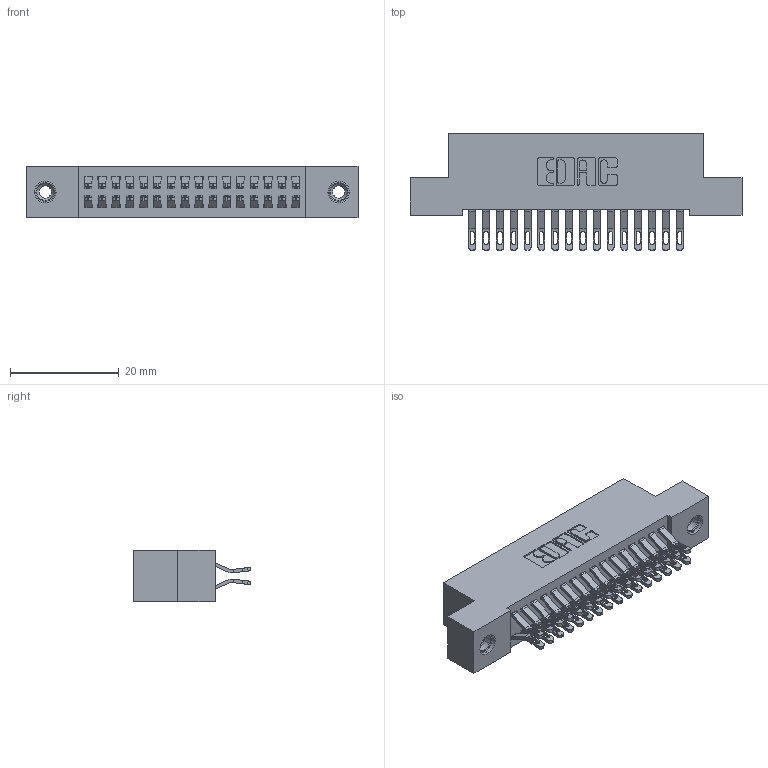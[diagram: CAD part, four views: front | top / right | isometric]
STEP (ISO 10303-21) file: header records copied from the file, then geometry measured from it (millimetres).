
FILE_DESCRIPTION (( 'STEP AP203' ), '1' );
FILE_NAME ('342-032-555-208.STEP', '2018-08-11T17:15:33', ( '' ), ( '' ), 'SwSTEP 2.0', 'SolidWorks 2016', '' );
FILE_SCHEMA (( 'CONFIG_CONTROL_DESIGN' ));
Length unit declared in the file: inch
Products named in the file (4): 342 Part_TI; 345-292-001_555 Tail; 345-250-001_345-250-003-102; 342-032-555-208
Assembly tree (35 placements, depth 2):
  342-032-555-208
    342 Part_TI
    345-292-001_555 Tail  x32
    345-250-001_345-250-003-102  x2
Bounding box: 60.96 x 21.47 x 9.4 mm (x, y, z)
Volume: 5437.4 mm3; surface area: 8530 mm2
Topology: 35 solids, 35 shells, 2026 faces, 6291 edges, 4186 vertices
Faces by surface type: plane 1186, cylinder 824, cone 12, torus 4
Entity records: 15036 total; most frequent: CARTESIAN_POINT 2539, ORIENTED_EDGE 2438, DIRECTION 2217, EDGE_CURVE 1219, LINE 1051, VECTOR 1051, VERTEX_POINT 808, AXIS2_PLACEMENT_3D 583
